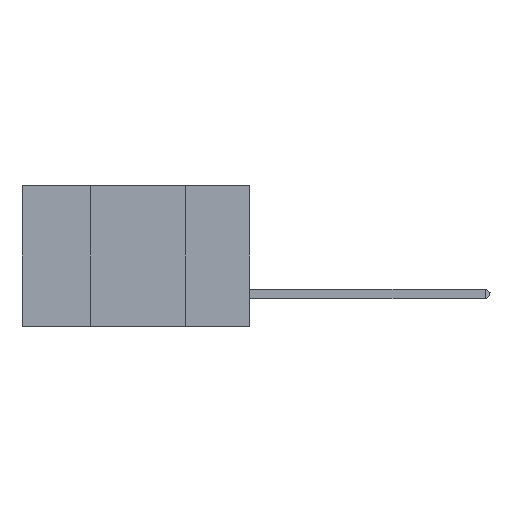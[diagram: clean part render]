
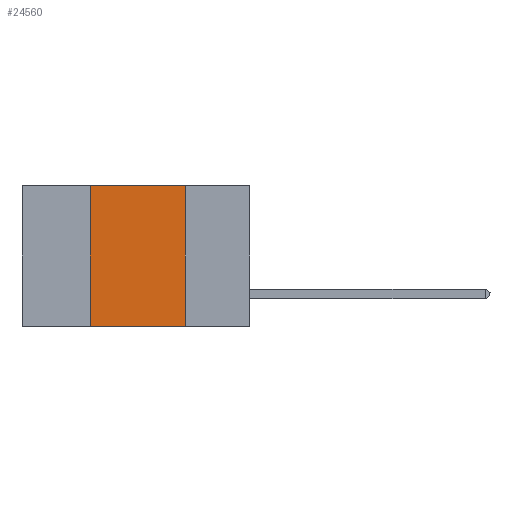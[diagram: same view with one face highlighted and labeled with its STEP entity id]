
A CAD part, left-side view. The second image highlights one B-rep face of the part: STEP entity #24560.
In plain terms, the highlighted planar face has unit normal (-1, 0, 0).
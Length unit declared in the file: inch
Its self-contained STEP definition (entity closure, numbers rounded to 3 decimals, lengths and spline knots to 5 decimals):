
#315 = VERTEX_POINT ( 'NONE', #23691 ) ;
#2112 = DIRECTION ( 'NONE',  ( 0., 0., -1. ) ) ;
#2174 = DIRECTION ( 'NONE',  ( 1., 0., 0. ) ) ;
#3448 = DIRECTION ( 'NONE',  ( 0., -1., 0. ) ) ;
#3956 = EDGE_CURVE ( 'NONE', #8658, #7555, #7943, .T. ) ;
#5103 = DIRECTION ( 'NONE',  ( 0., 0., 1. ) ) ;
#5873 = VECTOR ( 'NONE', #2112, 39.37008 ) ;
#6215 = VECTOR ( 'NONE', #7928, 39.37008 ) ;
#7097 = EDGE_LOOP ( 'NONE', ( #14406, #12316, #10640, #20844 ) ) ;
#7217 = CARTESIAN_POINT ( 'NONE',  ( 0., 0.17, -0.37 ) ) ;
#7555 = VERTEX_POINT ( 'NONE', #7217 ) ;
#7928 = DIRECTION ( 'NONE',  ( 0., -1., 0. ) ) ;
#7943 = LINE ( 'NONE', #20736, #14000 ) ;
#8567 = EDGE_CURVE ( 'NONE', #18766, #315, #10155, .T. ) ;
#8658 = VERTEX_POINT ( 'NONE', #24648 ) ;
#9152 = CARTESIAN_POINT ( 'NONE',  ( 0., 0.42, 0. ) ) ;
#9475 = EDGE_CURVE ( 'NONE', #315, #7555, #21317, .T. ) ;
#10155 = LINE ( 'NONE', #12970, #6215 ) ;
#10640 = ORIENTED_EDGE ( 'NONE', *, *, #14418, .F. ) ;
#11530 = CARTESIAN_POINT ( 'NONE',  ( 0., 0.17, 0. ) ) ;
#12316 = ORIENTED_EDGE ( 'NONE', *, *, #8567, .F. ) ;
#12970 = CARTESIAN_POINT ( 'NONE',  ( 0., 0.6, 0. ) ) ;
#13744 = PLANE ( 'NONE',  #16907 ) ;
#13825 = DIRECTION ( 'NONE',  ( 0., 0., -1. ) ) ;
#14000 = VECTOR ( 'NONE', #3448, 39.37008 ) ;
#14406 = ORIENTED_EDGE ( 'NONE', *, *, #9475, .F. ) ;
#14418 = EDGE_CURVE ( 'NONE', #8658, #18766, #18642, .T. ) ;
#16907 = AXIS2_PLACEMENT_3D ( 'NONE', #21300, #2174, #13825 ) ;
#18642 = LINE ( 'NONE', #9152, #19856 ) ;
#18766 = VERTEX_POINT ( 'NONE', #23969 ) ;
#19856 = VECTOR ( 'NONE', #5103, 39.37008 ) ;
#20736 = CARTESIAN_POINT ( 'NONE',  ( 0., 0.6, -0.37 ) ) ;
#20844 = ORIENTED_EDGE ( 'NONE', *, *, #3956, .T. ) ;
#21300 = CARTESIAN_POINT ( 'NONE',  ( 0., 0.6, 0. ) ) ;
#21317 = LINE ( 'NONE', #11530, #5873 ) ;
#23691 = CARTESIAN_POINT ( 'NONE',  ( 0., 0.17, 0. ) ) ;
#23969 = CARTESIAN_POINT ( 'NONE',  ( 0., 0.42, 0. ) ) ;
#24190 = FACE_OUTER_BOUND ( 'NONE', #7097, .T. ) ;
#24560 = ADVANCED_FACE ( 'NONE', ( #24190 ), #13744, .F. ) ;
#24648 = CARTESIAN_POINT ( 'NONE',  ( 0., 0.42, -0.37 ) ) ;
